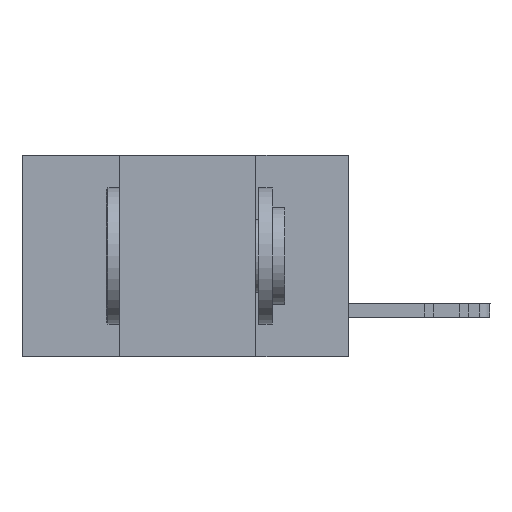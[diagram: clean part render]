
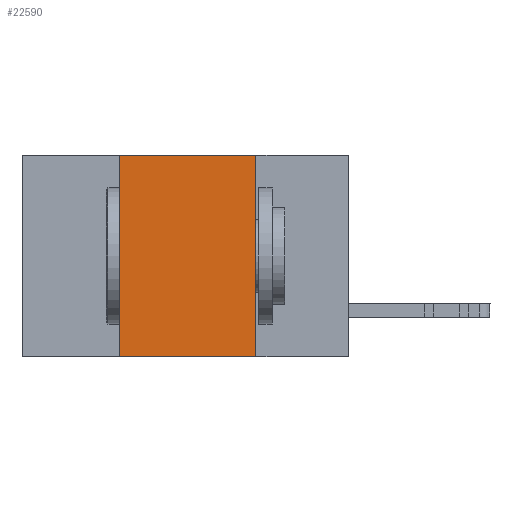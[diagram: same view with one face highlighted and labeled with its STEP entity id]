
A CAD part, left-side view. The second image highlights one B-rep face of the part: STEP entity #22590.
In plain terms, the highlighted planar face has unit normal (-1, 0, 0).
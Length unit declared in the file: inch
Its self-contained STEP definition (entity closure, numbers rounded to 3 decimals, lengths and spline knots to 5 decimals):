
#1111 = ORIENTED_EDGE ( 'NONE', *, *, #17612, .F. ) ;
#1493 = DIRECTION ( 'NONE',  ( 0., 0., -1. ) ) ;
#2707 = DIRECTION ( 'NONE',  ( 0., -1., 0. ) ) ;
#2811 = VERTEX_POINT ( 'NONE', #15882 ) ;
#2978 = ORIENTED_EDGE ( 'NONE', *, *, #14250, .F. ) ;
#3205 = CARTESIAN_POINT ( 'NONE',  ( 0., 0.42, -0.37 ) ) ;
#3557 = DIRECTION ( 'NONE',  ( 0., 0., 1. ) ) ;
#3885 = VECTOR ( 'NONE', #2707, 39.37008 ) ;
#3939 = VECTOR ( 'NONE', #3557, 39.37008 ) ;
#4669 = EDGE_LOOP ( 'NONE', ( #1111, #2978, #7177, #23781 ) ) ;
#4946 = PLANE ( 'NONE',  #16994 ) ;
#5074 = DIRECTION ( 'NONE',  ( 1., 0., 0. ) ) ;
#5637 = DIRECTION ( 'NONE',  ( 0., -1., 0. ) ) ;
#6105 = VECTOR ( 'NONE', #5637, 39.37008 ) ;
#7177 = ORIENTED_EDGE ( 'NONE', *, *, #13984, .F. ) ;
#7348 = CARTESIAN_POINT ( 'NONE',  ( 0., 0.6, 0. ) ) ;
#7473 = LINE ( 'NONE', #7348, #6105 ) ;
#8478 = VECTOR ( 'NONE', #1493, 39.37008 ) ;
#9073 = CARTESIAN_POINT ( 'NONE',  ( 0., 0.42, -0.37 ) ) ;
#9934 = VERTEX_POINT ( 'NONE', #10715 ) ;
#10243 = EDGE_CURVE ( 'NONE', #18317, #11540, #20517, .T. ) ;
#10715 = CARTESIAN_POINT ( 'NONE',  ( 0., 0.17, 0. ) ) ;
#11540 = VERTEX_POINT ( 'NONE', #16068 ) ;
#12940 = CARTESIAN_POINT ( 'NONE',  ( 0., 0.6, 0. ) ) ;
#13676 = LINE ( 'NONE', #17872, #8478 ) ;
#13984 = EDGE_CURVE ( 'NONE', #18317, #2811, #19163, .T. ) ;
#14250 = EDGE_CURVE ( 'NONE', #2811, #9934, #7473, .T. ) ;
#15882 = CARTESIAN_POINT ( 'NONE',  ( 0., 0.42, 0. ) ) ;
#16068 = CARTESIAN_POINT ( 'NONE',  ( 0., 0.17, -0.37 ) ) ;
#16994 = AXIS2_PLACEMENT_3D ( 'NONE', #12940, #5074, #22783 ) ;
#17612 = EDGE_CURVE ( 'NONE', #9934, #11540, #13676, .T. ) ;
#17872 = CARTESIAN_POINT ( 'NONE',  ( 0., 0.17, -0.37 ) ) ;
#18317 = VERTEX_POINT ( 'NONE', #3205 ) ;
#19163 = LINE ( 'NONE', #9073, #3939 ) ;
#20517 = LINE ( 'NONE', #22627, #3885 ) ;
#22590 = ADVANCED_FACE ( 'NONE', ( #25017 ), #4946, .F. ) ;
#22627 = CARTESIAN_POINT ( 'NONE',  ( 0., 0.6, -0.37 ) ) ;
#22783 = DIRECTION ( 'NONE',  ( 0., 0., -1. ) ) ;
#23781 = ORIENTED_EDGE ( 'NONE', *, *, #10243, .T. ) ;
#25017 = FACE_OUTER_BOUND ( 'NONE', #4669, .T. ) ;
